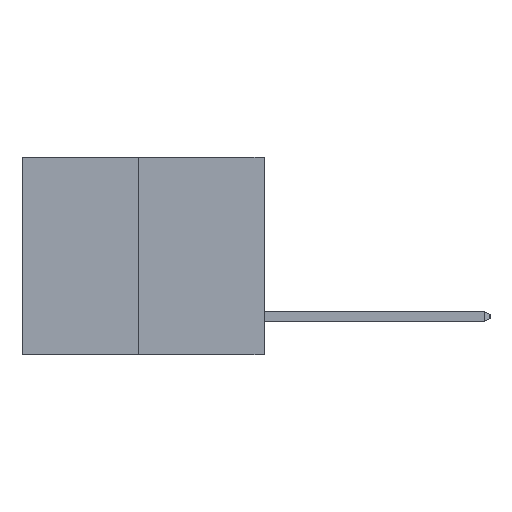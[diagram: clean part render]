
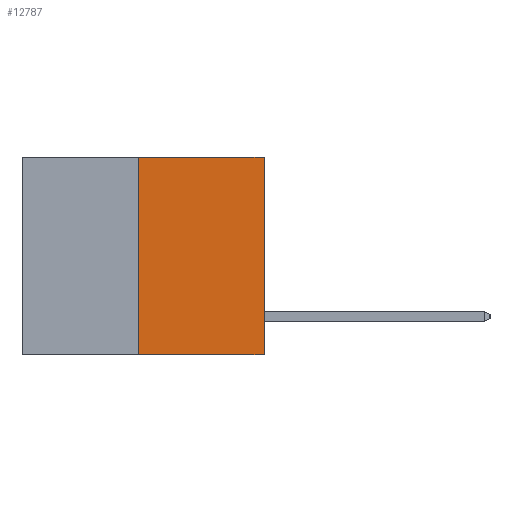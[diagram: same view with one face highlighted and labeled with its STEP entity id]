
A CAD part, left-side view. The second image highlights one B-rep face of the part: STEP entity #12787.
In plain terms, the highlighted planar face has unit normal (-1, 0, 0).
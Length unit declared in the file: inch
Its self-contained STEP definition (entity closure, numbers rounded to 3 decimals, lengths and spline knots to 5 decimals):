
#1148 = EDGE_CURVE ( 'NONE', #3150, #2880, #5151, .T. ) ;
#1384 = ORIENTED_EDGE ( 'NONE', *, *, #9094, .F. ) ;
#1484 = AXIS2_PLACEMENT_3D ( 'NONE', #12135, #14321, #2645 ) ;
#2267 = DIRECTION ( 'NONE',  ( 0., 0., 1. ) ) ;
#2386 = CARTESIAN_POINT ( 'NONE',  ( 0., 0., 0. ) ) ;
#2645 = DIRECTION ( 'NONE',  ( 0., 0., -1. ) ) ;
#2880 = VERTEX_POINT ( 'NONE', #3763 ) ;
#2905 = EDGE_LOOP ( 'NONE', ( #1384, #14240, #11186, #5631 ) ) ;
#3150 = VERTEX_POINT ( 'NONE', #5425 ) ;
#3273 = VERTEX_POINT ( 'NONE', #12626 ) ;
#3431 = VECTOR ( 'NONE', #5816, 39.37008 ) ;
#3763 = CARTESIAN_POINT ( 'NONE',  ( 0., 0., 0. ) ) ;
#4275 = VECTOR ( 'NONE', #5776, 39.37008 ) ;
#4993 = PLANE ( 'NONE',  #1484 ) ;
#5151 = LINE ( 'NONE', #2386, #9368 ) ;
#5425 = CARTESIAN_POINT ( 'NONE',  ( 0., 0., -0.49 ) ) ;
#5631 = ORIENTED_EDGE ( 'NONE', *, *, #9620, .F. ) ;
#5776 = DIRECTION ( 'NONE',  ( 0., -1., 0. ) ) ;
#5816 = DIRECTION ( 'NONE',  ( 0., -1., 0. ) ) ;
#6022 = DIRECTION ( 'NONE',  ( 0., 0., 1. ) ) ;
#6891 = LINE ( 'NONE', #10420, #7252 ) ;
#7252 = VECTOR ( 'NONE', #6022, 39.37008 ) ;
#7529 = CARTESIAN_POINT ( 'NONE',  ( 0., 0.312, 0. ) ) ;
#9094 = EDGE_CURVE ( 'NONE', #3273, #9285, #6891, .T. ) ;
#9285 = VERTEX_POINT ( 'NONE', #7529 ) ;
#9368 = VECTOR ( 'NONE', #2267, 39.37008 ) ;
#9620 = EDGE_CURVE ( 'NONE', #9285, #2880, #12465, .T. ) ;
#9925 = CARTESIAN_POINT ( 'NONE',  ( 0., 0.6, 0. ) ) ;
#10420 = CARTESIAN_POINT ( 'NONE',  ( 0., 0.312, -0.49 ) ) ;
#11186 = ORIENTED_EDGE ( 'NONE', *, *, #1148, .T. ) ;
#11501 = FACE_OUTER_BOUND ( 'NONE', #2905, .T. ) ;
#11588 = EDGE_CURVE ( 'NONE', #3273, #3150, #11780, .T. ) ;
#11780 = LINE ( 'NONE', #12960, #3431 ) ;
#12135 = CARTESIAN_POINT ( 'NONE',  ( 0., 0.6, 0. ) ) ;
#12465 = LINE ( 'NONE', #9925, #4275 ) ;
#12626 = CARTESIAN_POINT ( 'NONE',  ( 0., 0.312, -0.49 ) ) ;
#12787 = ADVANCED_FACE ( 'NONE', ( #11501 ), #4993, .F. ) ;
#12960 = CARTESIAN_POINT ( 'NONE',  ( 0., 0.6, -0.49 ) ) ;
#14240 = ORIENTED_EDGE ( 'NONE', *, *, #11588, .T. ) ;
#14321 = DIRECTION ( 'NONE',  ( 1., 0., 0. ) ) ;
